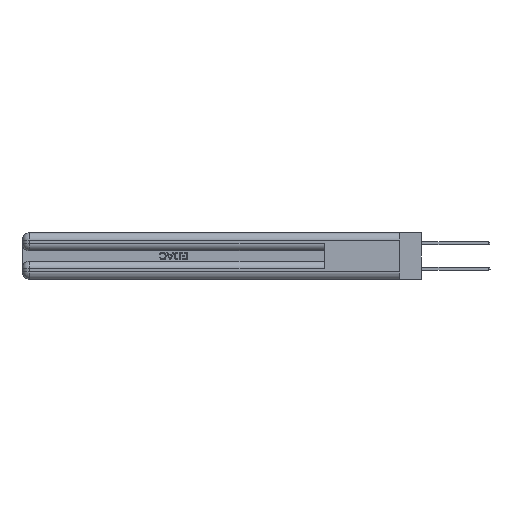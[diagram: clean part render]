
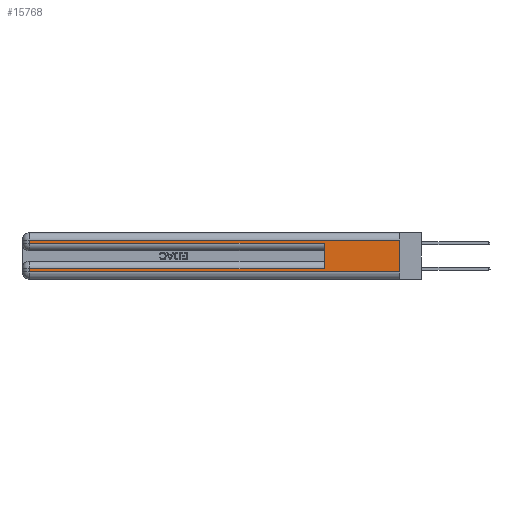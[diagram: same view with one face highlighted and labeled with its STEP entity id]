
A CAD part, left-side view. The second image highlights one B-rep face of the part: STEP entity #15768.
In plain terms, the highlighted planar face has unit normal (-1, 0, 0).
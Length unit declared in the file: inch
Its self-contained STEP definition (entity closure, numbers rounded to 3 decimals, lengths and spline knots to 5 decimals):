
#77 = VECTOR ( 'NONE', #643, 39.37008 ) ;
#218 = DIRECTION ( 'NONE',  ( 0., 0., -1. ) ) ;
#483 = DIRECTION ( 'NONE',  ( 0., 0., 1. ) ) ;
#643 = DIRECTION ( 'NONE',  ( 0., -1., 0. ) ) ;
#1536 = CARTESIAN_POINT ( 'NONE',  ( 0., 2.94, 0.31 ) ) ;
#1741 = EDGE_CURVE ( 'NONE', #15199, #39783, #42982, .T. ) ;
#2437 = CARTESIAN_POINT ( 'NONE',  ( 0., 0., 0.085 ) ) ;
#2718 = ORIENTED_EDGE ( 'NONE', *, *, #31339, .T. ) ;
#2848 = DIRECTION ( 'NONE',  ( 0., 0., -1. ) ) ;
#3008 = CARTESIAN_POINT ( 'NONE',  ( 0., 0., 0.37 ) ) ;
#5498 = EDGE_CURVE ( 'NONE', #43971, #25916, #25461, .T. ) ;
#7661 = DIRECTION ( 'NONE',  ( 0., -1., 0. ) ) ;
#8725 = LINE ( 'NONE', #33620, #11496 ) ;
#8842 = CARTESIAN_POINT ( 'NONE',  ( 0., 2.94, 0.085 ) ) ;
#11205 = DIRECTION ( 'NONE',  ( 0., 0., -1. ) ) ;
#11496 = VECTOR ( 'NONE', #483, 39.37008 ) ;
#11834 = ORIENTED_EDGE ( 'NONE', *, *, #1741, .T. ) ;
#12190 = CARTESIAN_POINT ( 'NONE',  ( 0., 2.94, 0.06 ) ) ;
#13197 = LINE ( 'NONE', #44124, #38716 ) ;
#13808 = CARTESIAN_POINT ( 'NONE',  ( 0., 0.6, 0.285 ) ) ;
#14059 = VECTOR ( 'NONE', #33816, 39.37008 ) ;
#14842 = CARTESIAN_POINT ( 'NONE',  ( 0., 0.6, 0.085 ) ) ;
#15199 = VERTEX_POINT ( 'NONE', #46496 ) ;
#15768 = ADVANCED_FACE ( 'NONE', ( #16802 ), #46231, .F. ) ;
#16802 = FACE_OUTER_BOUND ( 'NONE', #41653, .T. ) ;
#17533 = ORIENTED_EDGE ( 'NONE', *, *, #19880, .T. ) ;
#18185 = VECTOR ( 'NONE', #7661, 39.37008 ) ;
#19880 = EDGE_CURVE ( 'NONE', #39783, #39949, #28068, .T. ) ;
#20875 = EDGE_CURVE ( 'NONE', #32917, #43971, #13197, .T. ) ;
#21351 = EDGE_CURVE ( 'NONE', #15199, #25916, #30209, .T. ) ;
#22585 = AXIS2_PLACEMENT_3D ( 'NONE', #3008, #35460, #2848 ) ;
#22976 = EDGE_CURVE ( 'NONE', #46415, #32917, #23825, .T. ) ;
#23007 = ORIENTED_EDGE ( 'NONE', *, *, #21351, .F. ) ;
#23244 = VECTOR ( 'NONE', #27975, 39.37008 ) ;
#23825 = LINE ( 'NONE', #2437, #23244 ) ;
#24221 = ORIENTED_EDGE ( 'NONE', *, *, #5498, .T. ) ;
#24641 = CARTESIAN_POINT ( 'NONE',  ( 0., 0., 0.06 ) ) ;
#25461 = LINE ( 'NONE', #43569, #77 ) ;
#25614 = CARTESIAN_POINT ( 'NONE',  ( 0., 0., 0.37 ) ) ;
#25916 = VERTEX_POINT ( 'NONE', #24641 ) ;
#26673 = VERTEX_POINT ( 'NONE', #13808 ) ;
#26741 = LINE ( 'NONE', #28986, #18185 ) ;
#26876 = CARTESIAN_POINT ( 'NONE',  ( 0., 2.94, 0.285 ) ) ;
#27889 = ORIENTED_EDGE ( 'NONE', *, *, #20875, .T. ) ;
#27975 = DIRECTION ( 'NONE',  ( 0., 1., 0. ) ) ;
#28068 = LINE ( 'NONE', #32068, #35968 ) ;
#28986 = CARTESIAN_POINT ( 'NONE',  ( 0., 0., 0.285 ) ) ;
#30209 = LINE ( 'NONE', #25614, #38672 ) ;
#30351 = CARTESIAN_POINT ( 'NONE',  ( 0., 0., 0.31 ) ) ;
#30666 = EDGE_CURVE ( 'NONE', #46415, #26673, #8725, .T. ) ;
#31339 = EDGE_CURVE ( 'NONE', #39949, #26673, #26741, .T. ) ;
#32068 = CARTESIAN_POINT ( 'NONE',  ( 0., 2.94, 0.37 ) ) ;
#32917 = VERTEX_POINT ( 'NONE', #8842 ) ;
#33620 = CARTESIAN_POINT ( 'NONE',  ( 0., 0.6, 0.145 ) ) ;
#33816 = DIRECTION ( 'NONE',  ( 0., 1., 0. ) ) ;
#34604 = ORIENTED_EDGE ( 'NONE', *, *, #22976, .T. ) ;
#35460 = DIRECTION ( 'NONE',  ( 1., 0., 0. ) ) ;
#35968 = VECTOR ( 'NONE', #40346, 39.37008 ) ;
#38672 = VECTOR ( 'NONE', #218, 39.37008 ) ;
#38716 = VECTOR ( 'NONE', #11205, 39.37008 ) ;
#39783 = VERTEX_POINT ( 'NONE', #1536 ) ;
#39949 = VERTEX_POINT ( 'NONE', #26876 ) ;
#40346 = DIRECTION ( 'NONE',  ( 0., 0., -1. ) ) ;
#41653 = EDGE_LOOP ( 'NONE', ( #23007, #11834, #17533, #2718, #43272, #34604, #27889, #24221 ) ) ;
#42982 = LINE ( 'NONE', #30351, #14059 ) ;
#43272 = ORIENTED_EDGE ( 'NONE', *, *, #30666, .F. ) ;
#43569 = CARTESIAN_POINT ( 'NONE',  ( 0., 0., 0.06 ) ) ;
#43971 = VERTEX_POINT ( 'NONE', #12190 ) ;
#44124 = CARTESIAN_POINT ( 'NONE',  ( 0., 2.94, 0.37 ) ) ;
#46231 = PLANE ( 'NONE',  #22585 ) ;
#46415 = VERTEX_POINT ( 'NONE', #14842 ) ;
#46496 = CARTESIAN_POINT ( 'NONE',  ( 0., 0., 0.31 ) ) ;
